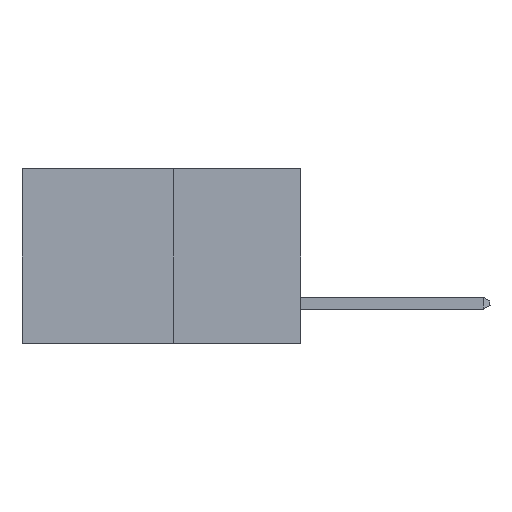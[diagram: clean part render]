
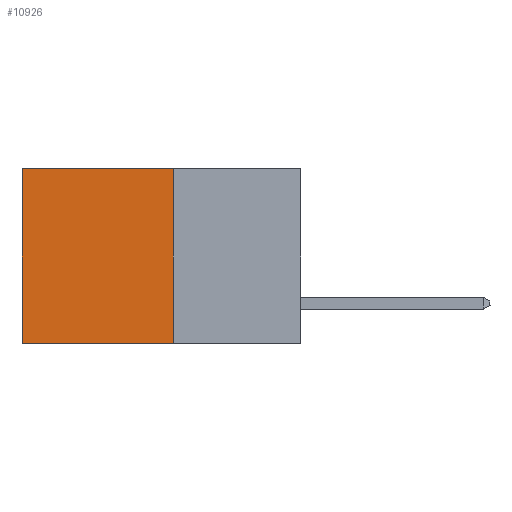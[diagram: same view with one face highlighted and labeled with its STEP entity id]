
A CAD part, left-side view. The second image highlights one B-rep face of the part: STEP entity #10926.
In plain terms, the highlighted planar face has unit normal (-1, 0, 0).
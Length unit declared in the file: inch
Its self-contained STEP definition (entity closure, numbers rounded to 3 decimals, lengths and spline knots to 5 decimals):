
#215 = VECTOR ( 'NONE', #2596, 39.37008 ) ;
#426 = EDGE_LOOP ( 'NONE', ( #9277, #10958, #14895, #3757 ) ) ;
#968 = EDGE_CURVE ( 'NONE', #8705, #18042, #16421, .T. ) ;
#1487 = VERTEX_POINT ( 'NONE', #14715 ) ;
#1542 = CARTESIAN_POINT ( 'NONE',  ( 0.277, 0.27, -0.37 ) ) ;
#1887 = CARTESIAN_POINT ( 'NONE',  ( 0.277, 0.27, 0. ) ) ;
#2596 = DIRECTION ( 'NONE',  ( 0., 1., 0. ) ) ;
#3428 = LINE ( 'NONE', #9187, #15800 ) ;
#3439 = CARTESIAN_POINT ( 'NONE',  ( 0.277, 0.27, -0.37 ) ) ;
#3757 = ORIENTED_EDGE ( 'NONE', *, *, #6042, .T. ) ;
#4203 = CARTESIAN_POINT ( 'NONE',  ( 0.277, 0.27, 0. ) ) ;
#4387 = LINE ( 'NONE', #1887, #16757 ) ;
#4981 = VECTOR ( 'NONE', #5959, 39.37008 ) ;
#5959 = DIRECTION ( 'NONE',  ( 0., 0., -1. ) ) ;
#6042 = EDGE_CURVE ( 'NONE', #20937, #1487, #4387, .T. ) ;
#8090 = DIRECTION ( 'NONE',  ( 0., 0., -1. ) ) ;
#8705 = VERTEX_POINT ( 'NONE', #11983 ) ;
#9187 = CARTESIAN_POINT ( 'NONE',  ( 0.277, 0.59, -0.37 ) ) ;
#9277 = ORIENTED_EDGE ( 'NONE', *, *, #20925, .T. ) ;
#9798 = LINE ( 'NONE', #17220, #4981 ) ;
#10807 = DIRECTION ( 'NONE',  ( 0., 0., -1. ) ) ;
#10926 = ADVANCED_FACE ( 'NONE', ( #11051 ), #16101, .F. ) ;
#10958 = ORIENTED_EDGE ( 'NONE', *, *, #968, .F. ) ;
#11051 = FACE_OUTER_BOUND ( 'NONE', #426, .T. ) ;
#11396 = AXIS2_PLACEMENT_3D ( 'NONE', #1542, #17743, #8090 ) ;
#11983 = CARTESIAN_POINT ( 'NONE',  ( 0.277, 0.27, -0.37 ) ) ;
#14715 = CARTESIAN_POINT ( 'NONE',  ( 0.277, 0.59, 0. ) ) ;
#14825 = DIRECTION ( 'NONE',  ( 0., 1., 0. ) ) ;
#14895 = ORIENTED_EDGE ( 'NONE', *, *, #19378, .F. ) ;
#15163 = CARTESIAN_POINT ( 'NONE',  ( 0.277, 0.59, -0.37 ) ) ;
#15800 = VECTOR ( 'NONE', #10807, 39.37008 ) ;
#16101 = PLANE ( 'NONE',  #11396 ) ;
#16421 = LINE ( 'NONE', #3439, #215 ) ;
#16757 = VECTOR ( 'NONE', #14825, 39.37008 ) ;
#17220 = CARTESIAN_POINT ( 'NONE',  ( 0.277, 0.27, -0.37 ) ) ;
#17743 = DIRECTION ( 'NONE',  ( 1., 0., 0. ) ) ;
#18042 = VERTEX_POINT ( 'NONE', #15163 ) ;
#19378 = EDGE_CURVE ( 'NONE', #20937, #8705, #9798, .T. ) ;
#20925 = EDGE_CURVE ( 'NONE', #1487, #18042, #3428, .T. ) ;
#20937 = VERTEX_POINT ( 'NONE', #4203 ) ;
